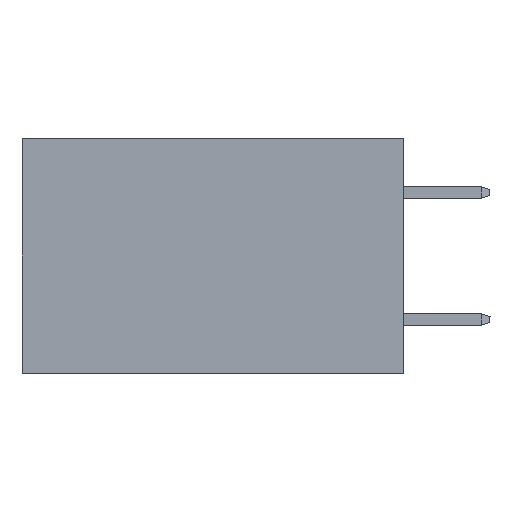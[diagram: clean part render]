
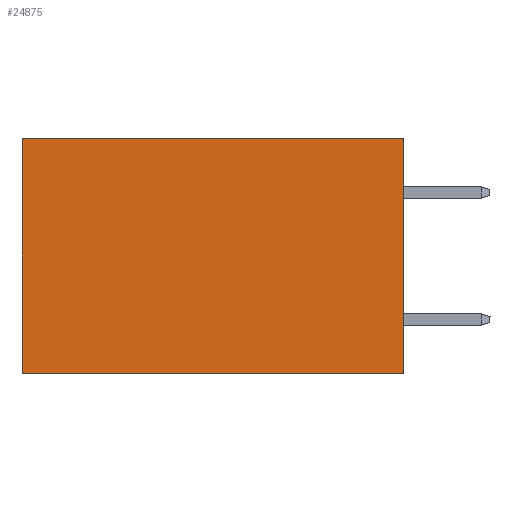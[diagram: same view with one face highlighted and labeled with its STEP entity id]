
A CAD part, left-side view. The second image highlights one B-rep face of the part: STEP entity #24875.
In plain terms, the highlighted planar face has unit normal (-1, 0, 0).
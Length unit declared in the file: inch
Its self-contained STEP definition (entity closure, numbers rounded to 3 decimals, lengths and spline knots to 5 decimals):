
#92 = PLANE ( 'NONE',  #4605 ) ;
#143 = LINE ( 'NONE', #11445, #24522 ) ;
#689 = CARTESIAN_POINT ( 'NONE',  ( 0.2875, 0.6, -0.37 ) ) ;
#1822 = DIRECTION ( 'NONE',  ( 1., 0., 0. ) ) ;
#3471 = DIRECTION ( 'NONE',  ( 0., 1., 0. ) ) ;
#3996 = CARTESIAN_POINT ( 'NONE',  ( 0.2875, 0., 0. ) ) ;
#4377 = EDGE_CURVE ( 'NONE', #24598, #17708, #18284, .T. ) ;
#4605 = AXIS2_PLACEMENT_3D ( 'NONE', #17681, #1822, #13407 ) ;
#5368 = LINE ( 'NONE', #14662, #9384 ) ;
#5678 = VECTOR ( 'NONE', #27618, 39.37008 ) ;
#8186 = CARTESIAN_POINT ( 'NONE',  ( 0.2875, 0., -0.37 ) ) ;
#9030 = VERTEX_POINT ( 'NONE', #23409 ) ;
#9384 = VECTOR ( 'NONE', #14525, 39.37008 ) ;
#9422 = DIRECTION ( 'NONE',  ( 0., 1., 0. ) ) ;
#11445 = CARTESIAN_POINT ( 'NONE',  ( 0.2875, 0., 0. ) ) ;
#13407 = DIRECTION ( 'NONE',  ( 0., 0., -1. ) ) ;
#14075 = EDGE_CURVE ( 'NONE', #24598, #9030, #143, .T. ) ;
#14525 = DIRECTION ( 'NONE',  ( 0., 0., -1. ) ) ;
#14634 = ORIENTED_EDGE ( 'NONE', *, *, #14075, .T. ) ;
#14662 = CARTESIAN_POINT ( 'NONE',  ( 0.2875, 0.6, 0. ) ) ;
#15363 = LINE ( 'NONE', #8186, #30124 ) ;
#15685 = ORIENTED_EDGE ( 'NONE', *, *, #15777, .T. ) ;
#15777 = EDGE_CURVE ( 'NONE', #9030, #24969, #5368, .T. ) ;
#15993 = ORIENTED_EDGE ( 'NONE', *, *, #4377, .F. ) ;
#17681 = CARTESIAN_POINT ( 'NONE',  ( 0.2875, 0., 0. ) ) ;
#17708 = VERTEX_POINT ( 'NONE', #17855 ) ;
#17855 = CARTESIAN_POINT ( 'NONE',  ( 0.2875, 0., -0.37 ) ) ;
#17986 = FACE_OUTER_BOUND ( 'NONE', #20317, .T. ) ;
#18284 = LINE ( 'NONE', #23144, #5678 ) ;
#20317 = EDGE_LOOP ( 'NONE', ( #15685, #29111, #15993, #14634 ) ) ;
#23144 = CARTESIAN_POINT ( 'NONE',  ( 0.2875, 0., 0. ) ) ;
#23409 = CARTESIAN_POINT ( 'NONE',  ( 0.2875, 0.6, 0. ) ) ;
#24522 = VECTOR ( 'NONE', #9422, 39.37008 ) ;
#24598 = VERTEX_POINT ( 'NONE', #3996 ) ;
#24875 = ADVANCED_FACE ( 'NONE', ( #17986 ), #92, .F. ) ;
#24969 = VERTEX_POINT ( 'NONE', #689 ) ;
#27618 = DIRECTION ( 'NONE',  ( 0., 0., -1. ) ) ;
#29111 = ORIENTED_EDGE ( 'NONE', *, *, #30112, .F. ) ;
#30112 = EDGE_CURVE ( 'NONE', #17708, #24969, #15363, .T. ) ;
#30124 = VECTOR ( 'NONE', #3471, 39.37008 ) ;
